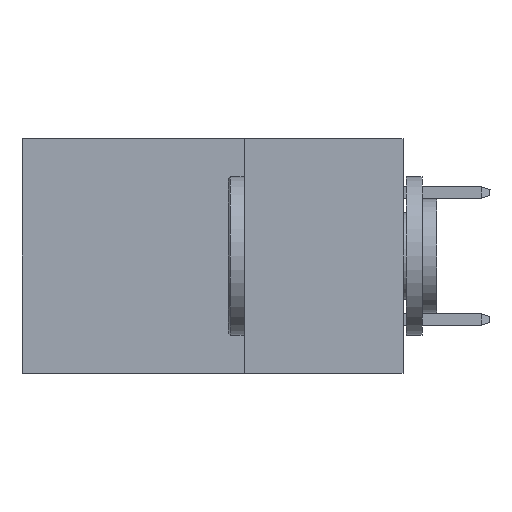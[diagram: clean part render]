
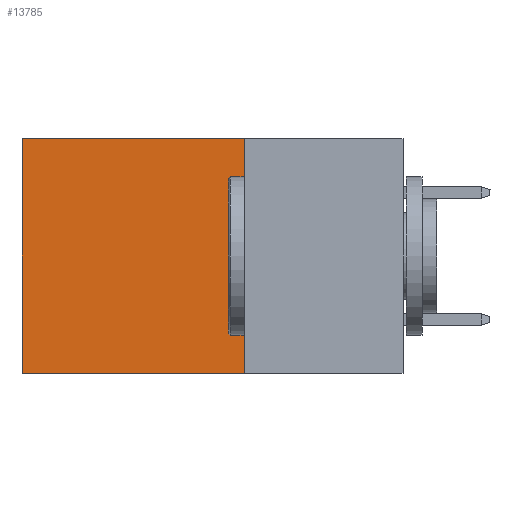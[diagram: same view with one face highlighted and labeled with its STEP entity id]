
A CAD part, left-side view. The second image highlights one B-rep face of the part: STEP entity #13785.
In plain terms, the highlighted planar face has unit normal (-1, 0, 0).
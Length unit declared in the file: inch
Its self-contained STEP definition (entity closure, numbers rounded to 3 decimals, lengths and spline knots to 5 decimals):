
#331 = VECTOR ( 'NONE', #18287, 39.37008 ) ;
#3023 = CARTESIAN_POINT ( 'NONE',  ( 0.2875, 0.6, 0. ) ) ;
#3051 = EDGE_CURVE ( 'NONE', #16668, #17164, #32999, .T. ) ;
#3525 = CARTESIAN_POINT ( 'NONE',  ( 0.2875, 0.25, 0. ) ) ;
#3771 = AXIS2_PLACEMENT_3D ( 'NONE', #3525, #9524, #15289 ) ;
#4649 = LINE ( 'NONE', #31355, #27572 ) ;
#5909 = CARTESIAN_POINT ( 'NONE',  ( 0.2875, 0.25, 0. ) ) ;
#7094 = VECTOR ( 'NONE', #21322, 39.37008 ) ;
#8183 = DIRECTION ( 'NONE',  ( 0., 0., -1. ) ) ;
#8975 = EDGE_CURVE ( 'NONE', #16944, #15229, #17628, .T. ) ;
#9310 = ORIENTED_EDGE ( 'NONE', *, *, #32948, .T. ) ;
#9524 = DIRECTION ( 'NONE',  ( 1., 0., 0. ) ) ;
#13785 = ADVANCED_FACE ( 'NONE', ( #29858 ), #18420, .F. ) ;
#14154 = CARTESIAN_POINT ( 'NONE',  ( 0.2875, 0.6, -0.37 ) ) ;
#14308 = DIRECTION ( 'NONE',  ( 0., 1., 0. ) ) ;
#15229 = VERTEX_POINT ( 'NONE', #30480 ) ;
#15289 = DIRECTION ( 'NONE',  ( 0., 0., -1. ) ) ;
#16668 = VERTEX_POINT ( 'NONE', #34739 ) ;
#16944 = VERTEX_POINT ( 'NONE', #22323 ) ;
#17058 = CARTESIAN_POINT ( 'NONE',  ( 0.2875, 0.25, 0. ) ) ;
#17164 = VERTEX_POINT ( 'NONE', #14154 ) ;
#17628 = LINE ( 'NONE', #17058, #30793 ) ;
#18287 = DIRECTION ( 'NONE',  ( 0., 0., -1. ) ) ;
#18420 = PLANE ( 'NONE',  #3771 ) ;
#18751 = ORIENTED_EDGE ( 'NONE', *, *, #3051, .T. ) ;
#20608 = LINE ( 'NONE', #5909, #7094 ) ;
#21322 = DIRECTION ( 'NONE',  ( 0., 1., 0. ) ) ;
#22323 = CARTESIAN_POINT ( 'NONE',  ( 0.2875, 0.25, 0. ) ) ;
#23542 = EDGE_CURVE ( 'NONE', #15229, #17164, #4649, .T. ) ;
#25837 = EDGE_LOOP ( 'NONE', ( #18751, #26517, #37401, #9310 ) ) ;
#26517 = ORIENTED_EDGE ( 'NONE', *, *, #23542, .F. ) ;
#27572 = VECTOR ( 'NONE', #14308, 39.37008 ) ;
#29858 = FACE_OUTER_BOUND ( 'NONE', #25837, .T. ) ;
#30480 = CARTESIAN_POINT ( 'NONE',  ( 0.2875, 0.25, -0.37 ) ) ;
#30793 = VECTOR ( 'NONE', #8183, 39.37008 ) ;
#31355 = CARTESIAN_POINT ( 'NONE',  ( 0.2875, 0.25, -0.37 ) ) ;
#32948 = EDGE_CURVE ( 'NONE', #16944, #16668, #20608, .T. ) ;
#32999 = LINE ( 'NONE', #3023, #331 ) ;
#34739 = CARTESIAN_POINT ( 'NONE',  ( 0.2875, 0.6, 0. ) ) ;
#37401 = ORIENTED_EDGE ( 'NONE', *, *, #8975, .F. ) ;
